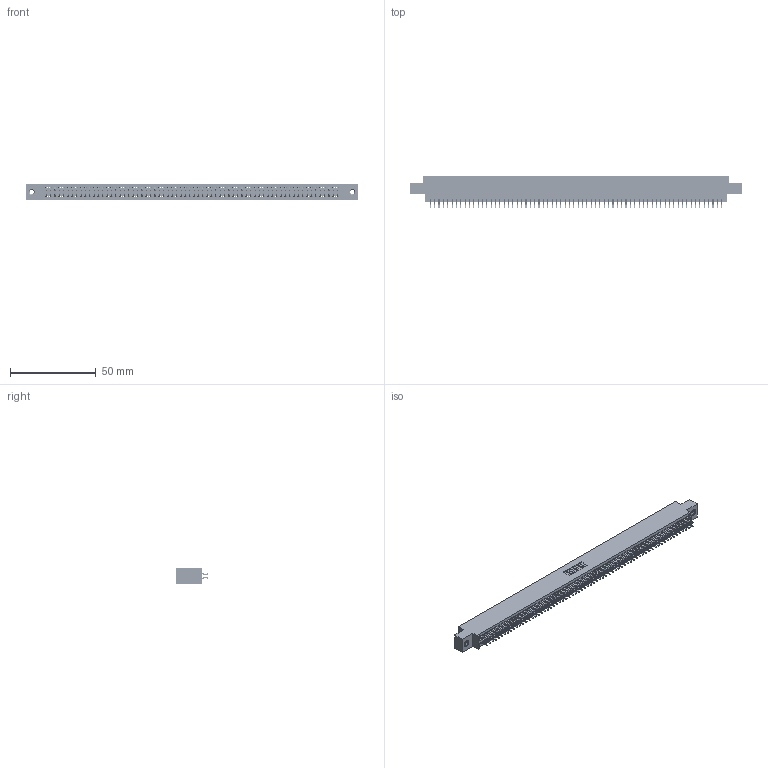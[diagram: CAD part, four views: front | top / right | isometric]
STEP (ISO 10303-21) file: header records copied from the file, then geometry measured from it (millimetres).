
FILE_DESCRIPTION (( 'STEP AP203' ), '1' );
FILE_NAME ('395-136-556-807.STEP', '2018-12-05T10:50:50', ( '' ), ( '' ), 'SwSTEP 2.0', 'SolidWorks 2016', '' );
FILE_SCHEMA (( 'CONFIG_CONTROL_DESIGN' ));
Length unit declared in the file: inch
Products named in the file (4): 345-250-001_345-250-005-103; 345-292-001_556 Tail; 345 Part_0.170 Offset - 0.156 Dia-TI; 395-136-556-807
Assembly tree (139 placements, depth 2):
  395-136-556-807
    345 Part_0.170 Offset - 0.156 Dia-TI
    345-292-001_556 Tail  x136
    345-250-001_345-250-005-103  x2
Bounding box: 193.93 x 19.24 x 9.4 mm (x, y, z)
Volume: 18947.5 mm3; surface area: 28563.5 mm2
Topology: 139 solids, 139 shells, 7806 faces, 23201 edges, 15278 vertices
Faces by surface type: plane 5148, cylinder 2642, cone 12, torus 4
Entity records: 51392 total; most frequent: CARTESIAN_POINT 8587, ORIENTED_EDGE 8502, DIRECTION 7553, EDGE_CURVE 4251, VECTOR 3819, LINE 3819, VERTEX_POINT 2828, AXIS2_PLACEMENT_3D 1867
